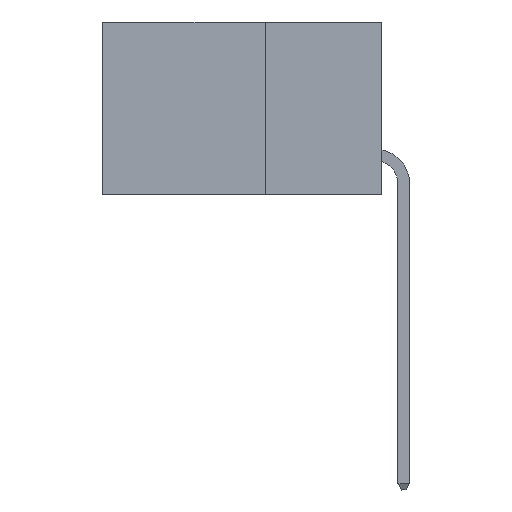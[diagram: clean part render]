
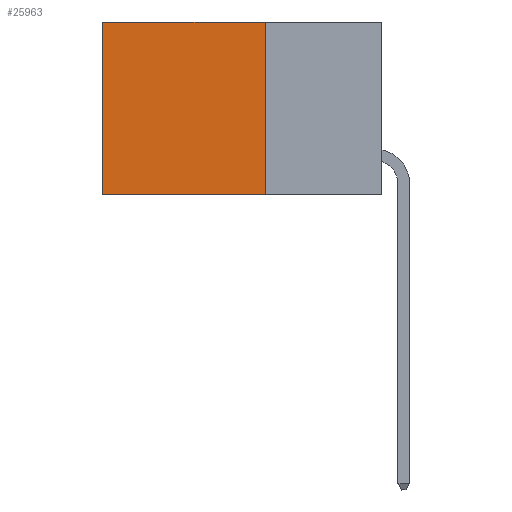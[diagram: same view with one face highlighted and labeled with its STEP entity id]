
A CAD part, left-side view. The second image highlights one B-rep face of the part: STEP entity #25963.
In plain terms, the highlighted planar face has unit normal (-1, 0, 0).
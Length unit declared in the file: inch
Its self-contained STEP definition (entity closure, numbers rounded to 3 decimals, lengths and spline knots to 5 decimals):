
#1252 = CARTESIAN_POINT ( 'NONE',  ( 0.2875, 0.25, -0.37 ) ) ;
#3859 = CARTESIAN_POINT ( 'NONE',  ( 0.2875, 0.25, 0. ) ) ;
#4721 = CARTESIAN_POINT ( 'NONE',  ( 0.2875, 0.6, 0. ) ) ;
#5354 = ORIENTED_EDGE ( 'NONE', *, *, #26671, .T. ) ;
#6394 = CARTESIAN_POINT ( 'NONE',  ( 0.2875, 0.25, 0. ) ) ;
#7690 = ORIENTED_EDGE ( 'NONE', *, *, #39039, .F. ) ;
#8623 = CARTESIAN_POINT ( 'NONE',  ( 0.2875, 0.25, 0. ) ) ;
#9099 = VECTOR ( 'NONE', #40144, 39.37008 ) ;
#11166 = DIRECTION ( 'NONE',  ( 0., 0., -1. ) ) ;
#14853 = LINE ( 'NONE', #1252, #9099 ) ;
#15210 = LINE ( 'NONE', #40301, #33324 ) ;
#16483 = ORIENTED_EDGE ( 'NONE', *, *, #34001, .T. ) ;
#16689 = VERTEX_POINT ( 'NONE', #4721 ) ;
#16864 = DIRECTION ( 'NONE',  ( 0., 1., 0. ) ) ;
#17401 = VECTOR ( 'NONE', #16864, 39.37008 ) ;
#17564 = CARTESIAN_POINT ( 'NONE',  ( 0.2875, 0.25, 0. ) ) ;
#18607 = VERTEX_POINT ( 'NONE', #33179 ) ;
#18839 = FACE_OUTER_BOUND ( 'NONE', #23540, .T. ) ;
#19092 = VECTOR ( 'NONE', #38302, 39.37008 ) ;
#21397 = PLANE ( 'NONE',  #34962 ) ;
#23540 = EDGE_LOOP ( 'NONE', ( #16483, #7690, #24939, #5354 ) ) ;
#23650 = LINE ( 'NONE', #3859, #17401 ) ;
#24939 = ORIENTED_EDGE ( 'NONE', *, *, #34431, .F. ) ;
#25963 = ADVANCED_FACE ( 'NONE', ( #18839 ), #21397, .F. ) ;
#26671 = EDGE_CURVE ( 'NONE', #32695, #16689, #23650, .T. ) ;
#31184 = DIRECTION ( 'NONE',  ( 0., 0., -1. ) ) ;
#32695 = VERTEX_POINT ( 'NONE', #17564 ) ;
#33179 = CARTESIAN_POINT ( 'NONE',  ( 0.2875, 0.25, -0.37 ) ) ;
#33324 = VECTOR ( 'NONE', #11166, 39.37008 ) ;
#33990 = CARTESIAN_POINT ( 'NONE',  ( 0.2875, 0.6, -0.37 ) ) ;
#34001 = EDGE_CURVE ( 'NONE', #16689, #38962, #15210, .T. ) ;
#34363 = DIRECTION ( 'NONE',  ( 1., 0., 0. ) ) ;
#34431 = EDGE_CURVE ( 'NONE', #32695, #18607, #38519, .T. ) ;
#34962 = AXIS2_PLACEMENT_3D ( 'NONE', #8623, #34363, #31184 ) ;
#38302 = DIRECTION ( 'NONE',  ( 0., 0., -1. ) ) ;
#38519 = LINE ( 'NONE', #6394, #19092 ) ;
#38962 = VERTEX_POINT ( 'NONE', #33990 ) ;
#39039 = EDGE_CURVE ( 'NONE', #18607, #38962, #14853, .T. ) ;
#40144 = DIRECTION ( 'NONE',  ( 0., 1., 0. ) ) ;
#40301 = CARTESIAN_POINT ( 'NONE',  ( 0.2875, 0.6, 0. ) ) ;
